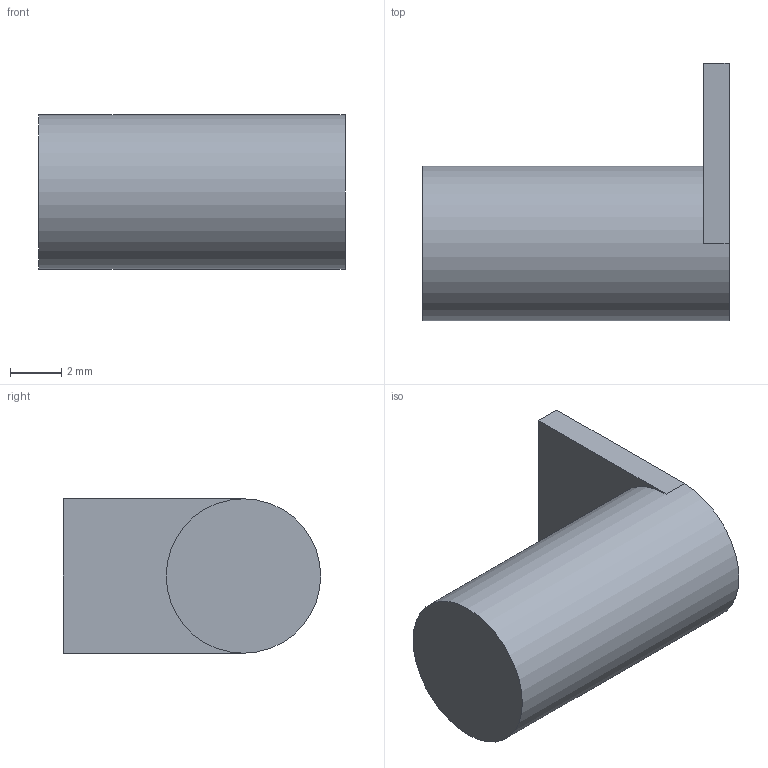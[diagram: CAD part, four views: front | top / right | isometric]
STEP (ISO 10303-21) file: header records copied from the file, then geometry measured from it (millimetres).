
FILE_DESCRIPTION((''),'2;1');
FILE_NAME('PM522SearPin2.stp','2015-10-01T18:17:18',('JamesRPatrick'),(''),'Autodesk Inventor 2012','Autodesk Inventor 2012','');
FILE_SCHEMA(('AUTOMOTIVE_DESIGN { 1 0 10303 214 1 1 1 1 }'));
Length unit declared in the file: millimetre
Products named in the file (1): PM522SearPin2
Bounding box: 11.9 x 10 x 6 mm (x, y, z)
Volume: 364.3 mm3; surface area: 347.2 mm2
Topology: 1 solids, 1 shells, 7 faces, 15 edges, 10 vertices
Faces by surface type: plane 6, cylinder 1
Full cylindrical faces by diameter (mm): 6 x1
Entity records: 204 total; most frequent: DIRECTION 32, CARTESIAN_POINT 30, ORIENTED_EDGE 26, EDGE_CURVE 13, AXIS2_PLACEMENT_3D 11, VECTOR 10, LINE 10, VERTEX_POINT 9
